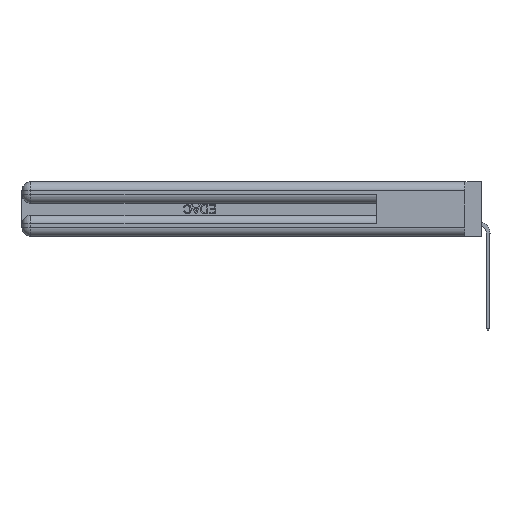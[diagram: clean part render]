
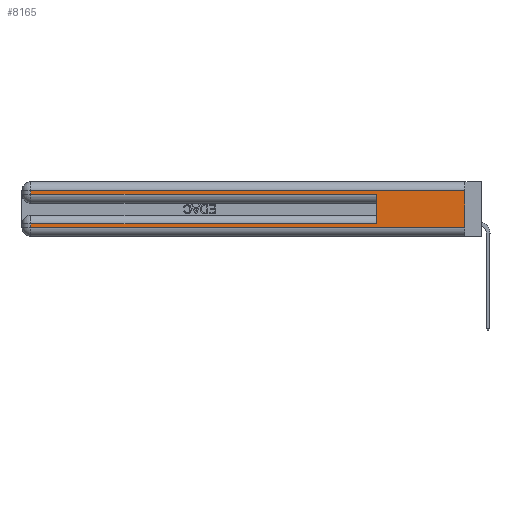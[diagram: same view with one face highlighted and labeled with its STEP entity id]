
A CAD part, left-side view. The second image highlights one B-rep face of the part: STEP entity #8165.
In plain terms, the highlighted planar face has unit normal (-1, 0, 0).
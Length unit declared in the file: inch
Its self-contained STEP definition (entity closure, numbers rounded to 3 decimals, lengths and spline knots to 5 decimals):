
#9 = VECTOR ( 'NONE', #10840, 39.37008 ) ;
#966 = ORIENTED_EDGE ( 'NONE', *, *, #41291, .T. ) ;
#981 = DIRECTION ( 'NONE',  ( 0., 0., -1. ) ) ;
#2740 = DIRECTION ( 'NONE',  ( 0., 0., 1. ) ) ;
#4707 = VERTEX_POINT ( 'NONE', #15168 ) ;
#6683 = VECTOR ( 'NONE', #35939, 39.37008 ) ;
#6771 = VERTEX_POINT ( 'NONE', #9363 ) ;
#8165 = ADVANCED_FACE ( 'NONE', ( #34671 ), #25389, .F. ) ;
#9363 = CARTESIAN_POINT ( 'NONE',  ( 0., 2.94, 0.285 ) ) ;
#10840 = DIRECTION ( 'NONE',  ( 0., 1., 0. ) ) ;
#11245 = EDGE_CURVE ( 'NONE', #42039, #6771, #13855, .T. ) ;
#11330 = CARTESIAN_POINT ( 'NONE',  ( 0., 0., 0.37 ) ) ;
#13308 = ORIENTED_EDGE ( 'NONE', *, *, #29042, .T. ) ;
#13437 = VERTEX_POINT ( 'NONE', #49945 ) ;
#13855 = LINE ( 'NONE', #25468, #24693 ) ;
#14693 = EDGE_LOOP ( 'NONE', ( #21741, #47786, #33349, #966, #47870, #16748, #13308, #43117 ) ) ;
#15168 = CARTESIAN_POINT ( 'NONE',  ( 0., 0., 0.31 ) ) ;
#15784 = CARTESIAN_POINT ( 'NONE',  ( 0., 0., 0.285 ) ) ;
#16482 = CARTESIAN_POINT ( 'NONE',  ( 0., 2.94, 0.085 ) ) ;
#16748 = ORIENTED_EDGE ( 'NONE', *, *, #46759, .T. ) ;
#20015 = CARTESIAN_POINT ( 'NONE',  ( 0., 0.6, 0.085 ) ) ;
#21741 = ORIENTED_EDGE ( 'NONE', *, *, #48675, .F. ) ;
#22483 = EDGE_CURVE ( 'NONE', #39277, #52005, #25099, .T. ) ;
#24355 = CARTESIAN_POINT ( 'NONE',  ( 0., 0., 0.085 ) ) ;
#24527 = LINE ( 'NONE', #44256, #36505 ) ;
#24693 = VECTOR ( 'NONE', #981, 39.37008 ) ;
#25099 = LINE ( 'NONE', #28327, #53944 ) ;
#25277 = LINE ( 'NONE', #15784, #39966 ) ;
#25321 = CARTESIAN_POINT ( 'NONE',  ( 0., 0., 0.06 ) ) ;
#25335 = VERTEX_POINT ( 'NONE', #25321 ) ;
#25384 = EDGE_CURVE ( 'NONE', #4707, #42039, #24527, .T. ) ;
#25389 = PLANE ( 'NONE',  #54188 ) ;
#25468 = CARTESIAN_POINT ( 'NONE',  ( 0., 2.94, 0.37 ) ) ;
#28327 = CARTESIAN_POINT ( 'NONE',  ( 0., 0.6, 0.145 ) ) ;
#29042 = EDGE_CURVE ( 'NONE', #42086, #13437, #38805, .T. ) ;
#32103 = DIRECTION ( 'NONE',  ( 0., -1., 0. ) ) ;
#33349 = ORIENTED_EDGE ( 'NONE', *, *, #11245, .T. ) ;
#33491 = CARTESIAN_POINT ( 'NONE',  ( 0., 2.94, 0.31 ) ) ;
#34671 = FACE_OUTER_BOUND ( 'NONE', #14693, .T. ) ;
#34998 = CARTESIAN_POINT ( 'NONE',  ( 0., 2.94, 0.37 ) ) ;
#35044 = EDGE_CURVE ( 'NONE', #13437, #25335, #48708, .T. ) ;
#35691 = DIRECTION ( 'NONE',  ( 0., 0., -1. ) ) ;
#35939 = DIRECTION ( 'NONE',  ( 0., 0., -1. ) ) ;
#36287 = DIRECTION ( 'NONE',  ( 0., 1., 0. ) ) ;
#36505 = VECTOR ( 'NONE', #36287, 39.37008 ) ;
#37402 = DIRECTION ( 'NONE',  ( 0., 0., -1. ) ) ;
#38805 = LINE ( 'NONE', #34998, #6683 ) ;
#39277 = VERTEX_POINT ( 'NONE', #20015 ) ;
#39966 = VECTOR ( 'NONE', #50178, 39.37008 ) ;
#41291 = EDGE_CURVE ( 'NONE', #6771, #52005, #25277, .T. ) ;
#42039 = VERTEX_POINT ( 'NONE', #33491 ) ;
#42086 = VERTEX_POINT ( 'NONE', #16482 ) ;
#43117 = ORIENTED_EDGE ( 'NONE', *, *, #35044, .T. ) ;
#44256 = CARTESIAN_POINT ( 'NONE',  ( 0., 0., 0.31 ) ) ;
#46186 = VECTOR ( 'NONE', #37402, 39.37008 ) ;
#46759 = EDGE_CURVE ( 'NONE', #39277, #42086, #54339, .T. ) ;
#47786 = ORIENTED_EDGE ( 'NONE', *, *, #25384, .T. ) ;
#47869 = DIRECTION ( 'NONE',  ( 1., 0., 0. ) ) ;
#47870 = ORIENTED_EDGE ( 'NONE', *, *, #22483, .F. ) ;
#48120 = LINE ( 'NONE', #11330, #46186 ) ;
#48228 = CARTESIAN_POINT ( 'NONE',  ( 0., 0., 0.37 ) ) ;
#48675 = EDGE_CURVE ( 'NONE', #4707, #25335, #48120, .T. ) ;
#48682 = CARTESIAN_POINT ( 'NONE',  ( 0., 0., 0.06 ) ) ;
#48708 = LINE ( 'NONE', #48682, #50729 ) ;
#49945 = CARTESIAN_POINT ( 'NONE',  ( 0., 2.94, 0.06 ) ) ;
#50178 = DIRECTION ( 'NONE',  ( 0., -1., 0. ) ) ;
#50729 = VECTOR ( 'NONE', #32103, 39.37008 ) ;
#51861 = CARTESIAN_POINT ( 'NONE',  ( 0., 0.6, 0.285 ) ) ;
#52005 = VERTEX_POINT ( 'NONE', #51861 ) ;
#53944 = VECTOR ( 'NONE', #2740, 39.37008 ) ;
#54188 = AXIS2_PLACEMENT_3D ( 'NONE', #48228, #47869, #35691 ) ;
#54339 = LINE ( 'NONE', #24355, #9 ) ;
